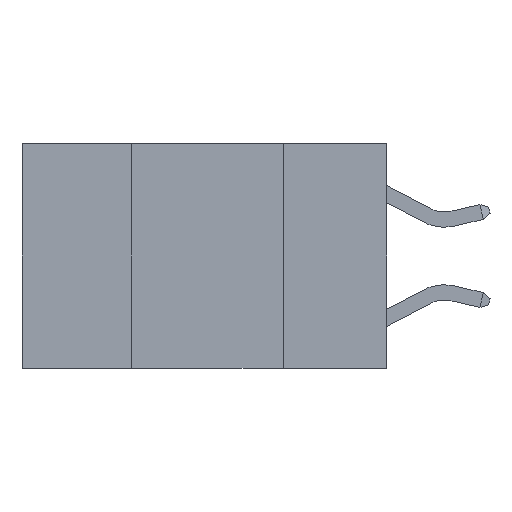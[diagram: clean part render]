
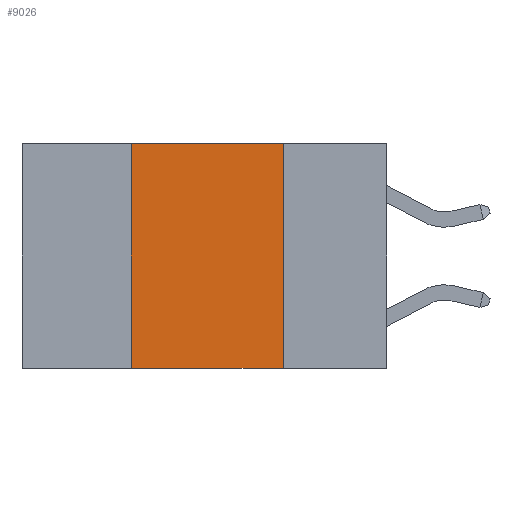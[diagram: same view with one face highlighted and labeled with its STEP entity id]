
A CAD part, left-side view. The second image highlights one B-rep face of the part: STEP entity #9026.
In plain terms, the highlighted planar face has unit normal (-1, 0, 0).
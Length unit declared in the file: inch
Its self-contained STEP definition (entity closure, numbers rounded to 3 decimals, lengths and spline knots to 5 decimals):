
#868 = DIRECTION ( 'NONE',  ( 0., 0., -1. ) ) ;
#1568 = EDGE_CURVE ( 'NONE', #13661, #12996, #14480, .T. ) ;
#2362 = CARTESIAN_POINT ( 'NONE',  ( 0., 0.17, 0. ) ) ;
#4161 = DIRECTION ( 'NONE',  ( 0., -1., 0. ) ) ;
#4891 = VECTOR ( 'NONE', #7639, 39.37008 ) ;
#5251 = EDGE_CURVE ( 'NONE', #24992, #12996, #25123, .T. ) ;
#5529 = CARTESIAN_POINT ( 'NONE',  ( 0., 0.42, -0.37 ) ) ;
#7209 = VECTOR ( 'NONE', #18507, 39.37008 ) ;
#7500 = LINE ( 'NONE', #16224, #7209 ) ;
#7639 = DIRECTION ( 'NONE',  ( 0., 0., -1. ) ) ;
#7830 = ORIENTED_EDGE ( 'NONE', *, *, #13496, .F. ) ;
#8449 = ORIENTED_EDGE ( 'NONE', *, *, #5251, .F. ) ;
#9026 = ADVANCED_FACE ( 'NONE', ( #11183 ), #13334, .F. ) ;
#10128 = VECTOR ( 'NONE', #4161, 39.37008 ) ;
#11183 = FACE_OUTER_BOUND ( 'NONE', #22507, .T. ) ;
#12996 = VERTEX_POINT ( 'NONE', #15569 ) ;
#13334 = PLANE ( 'NONE',  #23048 ) ;
#13414 = CARTESIAN_POINT ( 'NONE',  ( 0., 0.6, 0. ) ) ;
#13496 = EDGE_CURVE ( 'NONE', #17605, #24992, #17419, .T. ) ;
#13661 = VERTEX_POINT ( 'NONE', #5529 ) ;
#14480 = LINE ( 'NONE', #25953, #10128 ) ;
#15569 = CARTESIAN_POINT ( 'NONE',  ( 0., 0.17, -0.37 ) ) ;
#16224 = CARTESIAN_POINT ( 'NONE',  ( 0., 0.42, 0. ) ) ;
#17419 = LINE ( 'NONE', #13414, #18414 ) ;
#17605 = VERTEX_POINT ( 'NONE', #25143 ) ;
#18177 = CARTESIAN_POINT ( 'NONE',  ( 0., 0.6, 0. ) ) ;
#18414 = VECTOR ( 'NONE', #24607, 39.37008 ) ;
#18507 = DIRECTION ( 'NONE',  ( 0., 0., 1. ) ) ;
#20495 = CARTESIAN_POINT ( 'NONE',  ( 0., 0.17, 0. ) ) ;
#20821 = ORIENTED_EDGE ( 'NONE', *, *, #26539, .F. ) ;
#21651 = ORIENTED_EDGE ( 'NONE', *, *, #1568, .T. ) ;
#22507 = EDGE_LOOP ( 'NONE', ( #8449, #7830, #20821, #21651 ) ) ;
#23048 = AXIS2_PLACEMENT_3D ( 'NONE', #18177, #24808, #868 ) ;
#24607 = DIRECTION ( 'NONE',  ( 0., -1., 0. ) ) ;
#24808 = DIRECTION ( 'NONE',  ( 1., 0., 0. ) ) ;
#24992 = VERTEX_POINT ( 'NONE', #2362 ) ;
#25123 = LINE ( 'NONE', #20495, #4891 ) ;
#25143 = CARTESIAN_POINT ( 'NONE',  ( 0., 0.42, 0. ) ) ;
#25953 = CARTESIAN_POINT ( 'NONE',  ( 0., 0.6, -0.37 ) ) ;
#26539 = EDGE_CURVE ( 'NONE', #13661, #17605, #7500, .T. ) ;
